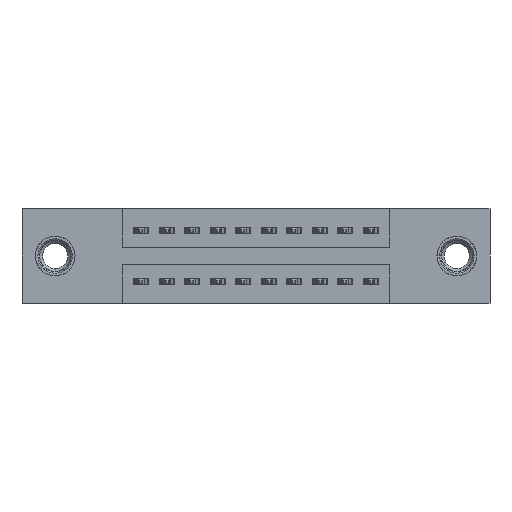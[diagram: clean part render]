
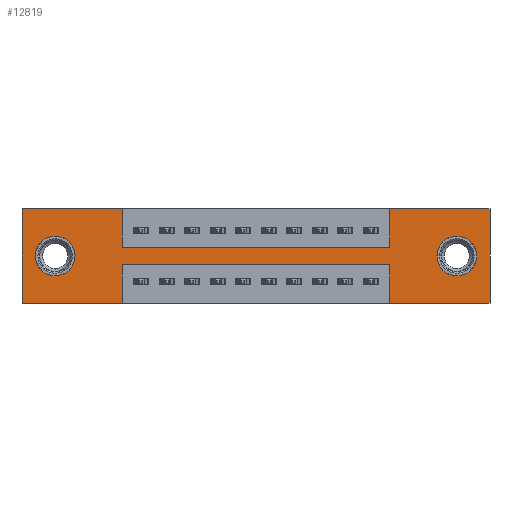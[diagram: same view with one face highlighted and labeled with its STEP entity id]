
A CAD part, front view. The second image highlights one B-rep face of the part: STEP entity #12819.
In plain terms, the highlighted planar face has unit normal (0, -1, 0).
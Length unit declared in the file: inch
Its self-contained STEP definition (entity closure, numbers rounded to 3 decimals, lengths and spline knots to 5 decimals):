
#30 = VERTEX_POINT ( 'NONE', #3242 ) ;
#59 = CARTESIAN_POINT ( 'NONE',  ( 0.3925, 0., -0.22 ) ) ;
#248 = AXIS2_PLACEMENT_3D ( 'NONE', #6496, #7623, #9703 ) ;
#302 = DIRECTION ( 'NONE',  ( 1., 0., 0. ) ) ;
#331 = DIRECTION ( 'NONE',  ( 0., 0., -1. ) ) ;
#566 = VERTEX_POINT ( 'NONE', #10634 ) ;
#666 = CARTESIAN_POINT ( 'NONE',  ( 1.4425, 0., -0.22 ) ) ;
#768 = CARTESIAN_POINT ( 'NONE',  ( 1.705, 0., -0.263 ) ) ;
#866 = VECTOR ( 'NONE', #12564, 39.37008 ) ;
#971 = VECTOR ( 'NONE', #302, 39.37008 ) ;
#1288 = ORIENTED_EDGE ( 'NONE', *, *, #7208, .T. ) ;
#1349 = LINE ( 'NONE', #7168, #2638 ) ;
#1391 = CARTESIAN_POINT ( 'NONE',  ( 1.705, 0., -0.107 ) ) ;
#1407 = CIRCLE ( 'NONE', #9050, 0.078 ) ;
#1463 = ORIENTED_EDGE ( 'NONE', *, *, #11191, .T. ) ;
#1491 = CARTESIAN_POINT ( 'NONE',  ( 1.835, 0., -0.37 ) ) ;
#1596 = VECTOR ( 'NONE', #1783, 39.37008 ) ;
#1759 = VERTEX_POINT ( 'NONE', #6005 ) ;
#1777 = ORIENTED_EDGE ( 'NONE', *, *, #3313, .F. ) ;
#1783 = DIRECTION ( 'NONE',  ( 0., 0., -1. ) ) ;
#1889 = VECTOR ( 'NONE', #6349, 39.37008 ) ;
#1972 = VERTEX_POINT ( 'NONE', #6612 ) ;
#2000 = CARTESIAN_POINT ( 'NONE',  ( 0.3925, 0., -0.15 ) ) ;
#2026 = DIRECTION ( 'NONE',  ( 1., 0., 0. ) ) ;
#2055 = CARTESIAN_POINT ( 'NONE',  ( 1.4425, 0., -0.37 ) ) ;
#2445 = PLANE ( 'NONE',  #248 ) ;
#2548 = CARTESIAN_POINT ( 'NONE',  ( 0.13, 0., -0.185 ) ) ;
#2582 = LINE ( 'NONE', #8208, #12447 ) ;
#2638 = VECTOR ( 'NONE', #11324, 39.37008 ) ;
#2711 = CARTESIAN_POINT ( 'NONE',  ( 0.3925, 0., 0. ) ) ;
#2923 = CARTESIAN_POINT ( 'NONE',  ( 1.705, 0., -0.185 ) ) ;
#3242 = CARTESIAN_POINT ( 'NONE',  ( 1.835, 0., 0. ) ) ;
#3291 = VECTOR ( 'NONE', #10210, 39.37008 ) ;
#3313 = EDGE_CURVE ( 'NONE', #9965, #7366, #12605, .T. ) ;
#3384 = CARTESIAN_POINT ( 'NONE',  ( 1.4425, 0., -0.15 ) ) ;
#3455 = VERTEX_POINT ( 'NONE', #7944 ) ;
#3587 = LINE ( 'NONE', #5562, #8306 ) ;
#3644 = FACE_BOUND ( 'NONE', #12329, .T. ) ;
#3668 = VECTOR ( 'NONE', #12125, 39.37008 ) ;
#3699 = VERTEX_POINT ( 'NONE', #6859 ) ;
#3831 = ORIENTED_EDGE ( 'NONE', *, *, #12470, .T. ) ;
#3955 = LINE ( 'NONE', #8142, #12525 ) ;
#4165 = ORIENTED_EDGE ( 'NONE', *, *, #9699, .F. ) ;
#4507 = VERTEX_POINT ( 'NONE', #2711 ) ;
#4620 = DIRECTION ( 'NONE',  ( 0., 0., 1. ) ) ;
#4636 = ORIENTED_EDGE ( 'NONE', *, *, #7907, .F. ) ;
#4857 = ORIENTED_EDGE ( 'NONE', *, *, #9920, .F. ) ;
#4985 = LINE ( 'NONE', #11473, #1889 ) ;
#5130 = VERTEX_POINT ( 'NONE', #666 ) ;
#5186 = ORIENTED_EDGE ( 'NONE', *, *, #12388, .F. ) ;
#5192 = ORIENTED_EDGE ( 'NONE', *, *, #9303, .F. ) ;
#5194 = VECTOR ( 'NONE', #13081, 39.37008 ) ;
#5548 = EDGE_LOOP ( 'NONE', ( #9591, #7785, #4165, #9538, #11269, #4636, #5186, #1777, #5192, #7636, #9893, #4857 ) ) ;
#5552 = AXIS2_PLACEMENT_3D ( 'NONE', #11050, #8918, #10963 ) ;
#5562 = CARTESIAN_POINT ( 'NONE',  ( 0., 0., -0.37 ) ) ;
#5588 = EDGE_CURVE ( 'NONE', #10759, #3699, #1407, .T. ) ;
#5825 = VERTEX_POINT ( 'NONE', #768 ) ;
#5865 = CARTESIAN_POINT ( 'NONE',  ( 0., 0., -0.37 ) ) ;
#5972 = VERTEX_POINT ( 'NONE', #1491 ) ;
#6005 = CARTESIAN_POINT ( 'NONE',  ( 0.3925, 0., -0.37 ) ) ;
#6069 = CARTESIAN_POINT ( 'NONE',  ( 0.3925, 0., 0. ) ) ;
#6151 = AXIS2_PLACEMENT_3D ( 'NONE', #11728, #12635, #331 ) ;
#6190 = CARTESIAN_POINT ( 'NONE',  ( 1.835, 0., 0. ) ) ;
#6244 = DIRECTION ( 'NONE',  ( 0., 1., 0. ) ) ;
#6349 = DIRECTION ( 'NONE',  ( 0., 0., 1. ) ) ;
#6440 = LINE ( 'NONE', #12037, #3668 ) ;
#6496 = CARTESIAN_POINT ( 'NONE',  ( 0., 0., -0.37 ) ) ;
#6599 = DIRECTION ( 'NONE',  ( -1., 0., 0. ) ) ;
#6612 = CARTESIAN_POINT ( 'NONE',  ( 0., 0., 0. ) ) ;
#6859 = CARTESIAN_POINT ( 'NONE',  ( 0.13, 0., -0.263 ) ) ;
#6958 = VERTEX_POINT ( 'NONE', #2055 ) ;
#7147 = LINE ( 'NONE', #6069, #5194 ) ;
#7168 = CARTESIAN_POINT ( 'NONE',  ( 0., 0., 0. ) ) ;
#7187 = EDGE_CURVE ( 'NONE', #5972, #6958, #3955, .T. ) ;
#7208 = EDGE_CURVE ( 'NONE', #9928, #5825, #12177, .T. ) ;
#7366 = VERTEX_POINT ( 'NONE', #3384 ) ;
#7611 = CARTESIAN_POINT ( 'NONE',  ( 0.13, 0., -0.107 ) ) ;
#7623 = DIRECTION ( 'NONE',  ( 0., -1., 0. ) ) ;
#7636 = ORIENTED_EDGE ( 'NONE', *, *, #7715, .F. ) ;
#7715 = EDGE_CURVE ( 'NONE', #1972, #4507, #13138, .T. ) ;
#7785 = ORIENTED_EDGE ( 'NONE', *, *, #8036, .F. ) ;
#7886 = EDGE_CURVE ( 'NONE', #30, #5972, #9142, .T. ) ;
#7907 = EDGE_CURVE ( 'NONE', #3455, #30, #1349, .T. ) ;
#7944 = CARTESIAN_POINT ( 'NONE',  ( 1.4425, 0., 0. ) ) ;
#8036 = EDGE_CURVE ( 'NONE', #5130, #566, #12966, .T. ) ;
#8142 = CARTESIAN_POINT ( 'NONE',  ( 0., 0., -0.37 ) ) ;
#8208 = CARTESIAN_POINT ( 'NONE',  ( 1.4425, 0., -0.37 ) ) ;
#8306 = VECTOR ( 'NONE', #6599, 39.37008 ) ;
#8608 = VERTEX_POINT ( 'NONE', #5865 ) ;
#8918 = DIRECTION ( 'NONE',  ( 0., 1., 0. ) ) ;
#9013 = CARTESIAN_POINT ( 'NONE',  ( 0.3925, 0., -0.37 ) ) ;
#9050 = AXIS2_PLACEMENT_3D ( 'NONE', #2548, #9812, #4620 ) ;
#9142 = LINE ( 'NONE', #6190, #3291 ) ;
#9250 = DIRECTION ( 'NONE',  ( 0., 0., 1. ) ) ;
#9303 = EDGE_CURVE ( 'NONE', #4507, #9965, #7147, .T. ) ;
#9490 = DIRECTION ( 'NONE',  ( 0., 0., -1. ) ) ;
#9538 = ORIENTED_EDGE ( 'NONE', *, *, #7187, .F. ) ;
#9591 = ORIENTED_EDGE ( 'NONE', *, *, #10918, .F. ) ;
#9699 = EDGE_CURVE ( 'NONE', #6958, #5130, #2582, .T. ) ;
#9703 = DIRECTION ( 'NONE',  ( 0., 0., -1. ) ) ;
#9812 = DIRECTION ( 'NONE',  ( 0., 1., 0. ) ) ;
#9893 = ORIENTED_EDGE ( 'NONE', *, *, #11096, .F. ) ;
#9920 = EDGE_CURVE ( 'NONE', #1759, #8608, #3587, .T. ) ;
#9928 = VERTEX_POINT ( 'NONE', #1391 ) ;
#9965 = VERTEX_POINT ( 'NONE', #2000 ) ;
#10210 = DIRECTION ( 'NONE',  ( 0., 0., -1. ) ) ;
#10310 = DIRECTION ( 'NONE',  ( -1., 0., 0. ) ) ;
#10610 = FACE_OUTER_BOUND ( 'NONE', #5548, .T. ) ;
#10634 = CARTESIAN_POINT ( 'NONE',  ( 0.3925, 0., -0.22 ) ) ;
#10759 = VERTEX_POINT ( 'NONE', #7611 ) ;
#10868 = ORIENTED_EDGE ( 'NONE', *, *, #5588, .T. ) ;
#10918 = EDGE_CURVE ( 'NONE', #566, #1759, #12100, .T. ) ;
#10963 = DIRECTION ( 'NONE',  ( 0., 0., 1. ) ) ;
#10996 = EDGE_LOOP ( 'NONE', ( #1288, #1463 ) ) ;
#11050 = CARTESIAN_POINT ( 'NONE',  ( 0.13, 0., -0.185 ) ) ;
#11096 = EDGE_CURVE ( 'NONE', #8608, #1972, #4985, .T. ) ;
#11191 = EDGE_CURVE ( 'NONE', #5825, #9928, #11930, .T. ) ;
#11269 = ORIENTED_EDGE ( 'NONE', *, *, #7886, .F. ) ;
#11324 = DIRECTION ( 'NONE',  ( 1., 0., 0. ) ) ;
#11473 = CARTESIAN_POINT ( 'NONE',  ( 0., 0., 0. ) ) ;
#11651 = CARTESIAN_POINT ( 'NONE',  ( 0.3925, 0., -0.15 ) ) ;
#11728 = CARTESIAN_POINT ( 'NONE',  ( 1.705, 0., -0.185 ) ) ;
#11930 = CIRCLE ( 'NONE', #6151, 0.078 ) ;
#12037 = CARTESIAN_POINT ( 'NONE',  ( 1.4425, 0., 0. ) ) ;
#12100 = LINE ( 'NONE', #9013, #1596 ) ;
#12125 = DIRECTION ( 'NONE',  ( 0., 0., 1. ) ) ;
#12177 = CIRCLE ( 'NONE', #12231, 0.078 ) ;
#12231 = AXIS2_PLACEMENT_3D ( 'NONE', #2923, #6244, #9490 ) ;
#12284 = CARTESIAN_POINT ( 'NONE',  ( 0., 0., 0. ) ) ;
#12329 = EDGE_LOOP ( 'NONE', ( #10868, #3831 ) ) ;
#12388 = EDGE_CURVE ( 'NONE', #7366, #3455, #6440, .T. ) ;
#12447 = VECTOR ( 'NONE', #9250, 39.37008 ) ;
#12470 = EDGE_CURVE ( 'NONE', #3699, #10759, #12540, .T. ) ;
#12525 = VECTOR ( 'NONE', #10310, 39.37008 ) ;
#12540 = CIRCLE ( 'NONE', #5552, 0.078 ) ;
#12564 = DIRECTION ( 'NONE',  ( -1., 0., 0. ) ) ;
#12605 = LINE ( 'NONE', #11651, #971 ) ;
#12635 = DIRECTION ( 'NONE',  ( 0., 1., 0. ) ) ;
#12697 = VECTOR ( 'NONE', #2026, 39.37008 ) ;
#12819 = ADVANCED_FACE ( 'NONE', ( #13320, #3644, #10610 ), #2445, .T. ) ;
#12966 = LINE ( 'NONE', #59, #866 ) ;
#13081 = DIRECTION ( 'NONE',  ( 0., 0., -1. ) ) ;
#13138 = LINE ( 'NONE', #12284, #12697 ) ;
#13320 = FACE_BOUND ( 'NONE', #10996, .T. ) ;
